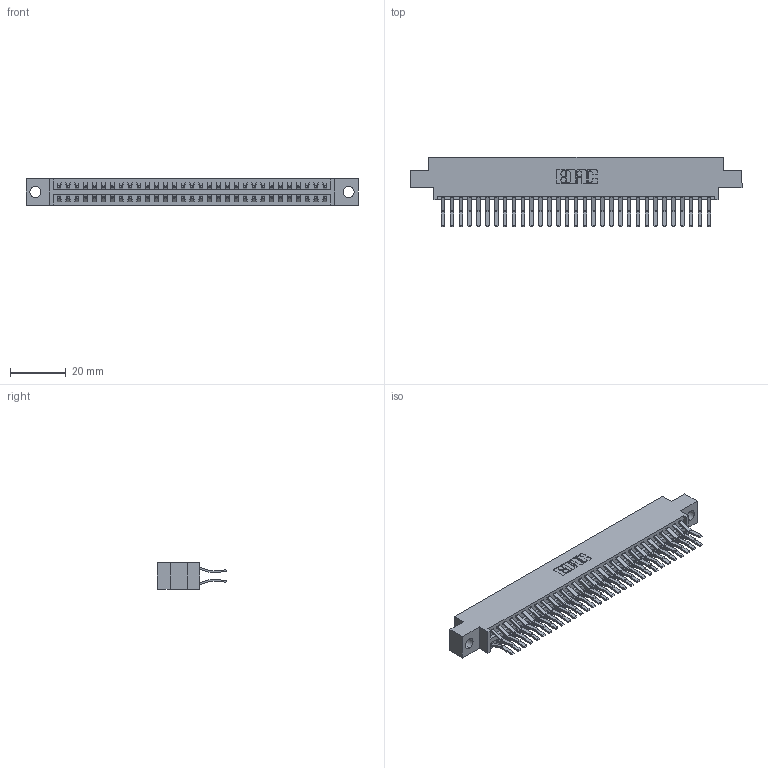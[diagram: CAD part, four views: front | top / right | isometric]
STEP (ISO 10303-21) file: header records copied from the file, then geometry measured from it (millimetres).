
FILE_DESCRIPTION (( 'STEP AP203' ), '1' );
FILE_NAME ('396-062-560-804.STEP', '2018-09-08T16:16:38', ( '' ), ( '' ), 'SwSTEP 2.0', 'SolidWorks 2016', '' );
FILE_SCHEMA (( 'CONFIG_CONTROL_DESIGN' ));
Length unit declared in the file: inch
Products named in the file (3): 346 Part_0.170 Offset - 0.156 Dia-TH; 345-292-001_560 Tail; 396-062-560-804
Assembly tree (63 placements, depth 2):
  396-062-560-804
    346 Part_0.170 Offset - 0.156 Dia-TH
    345-292-001_560 Tail  x62
Bounding box: 119 x 24.78 x 9.4 mm (x, y, z)
Volume: 11682.4 mm3; surface area: 16962.5 mm2
Topology: 63 solids, 63 shells, 3474 faces, 10323 edges, 6798 vertices
Faces by surface type: plane 2250, cylinder 1224
Entity records: 21935 total; most frequent: CARTESIAN_POINT 3632, ORIENTED_EDGE 3566, DIRECTION 3255, EDGE_CURVE 1783, VECTOR 1523, LINE 1523, VERTEX_POINT 1186, AXIS2_PLACEMENT_3D 866
